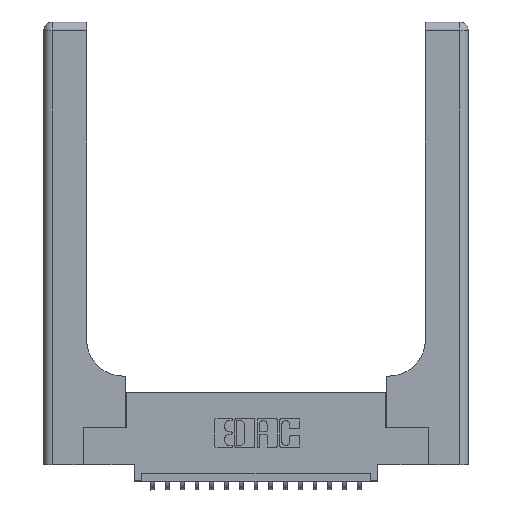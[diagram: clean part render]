
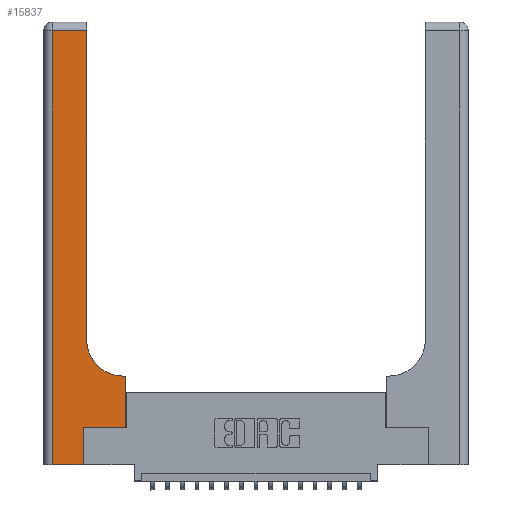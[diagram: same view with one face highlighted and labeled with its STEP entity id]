
A CAD part, top view. The second image highlights one B-rep face of the part: STEP entity #15837.
In plain terms, the highlighted planar face has unit normal (0, 0, 1).
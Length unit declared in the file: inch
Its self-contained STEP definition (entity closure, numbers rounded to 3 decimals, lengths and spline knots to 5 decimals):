
#398 = DIRECTION ( 'NONE',  ( -1., 0., 0. ) ) ;
#473 = EDGE_CURVE ( 'NONE', #16439, #4550, #7650, .T. ) ;
#478 = ORIENTED_EDGE ( 'NONE', *, *, #10949, .T. ) ;
#588 = VECTOR ( 'NONE', #18240, 39.37008 ) ;
#759 = VECTOR ( 'NONE', #15588, 39.37008 ) ;
#807 = ORIENTED_EDGE ( 'NONE', *, *, #1249, .T. ) ;
#1249 = EDGE_CURVE ( 'NONE', #12366, #1956, #19674, .T. ) ;
#1771 = AXIS2_PLACEMENT_3D ( 'NONE', #9812, #11354, #17633 ) ;
#1929 = CARTESIAN_POINT ( 'NONE',  ( 0.2915, 3., 0.37 ) ) ;
#1956 = VERTEX_POINT ( 'NONE', #12227 ) ;
#2508 = CARTESIAN_POINT ( 'NONE',  ( 0.5415, 0.6, 0.37 ) ) ;
#2827 = EDGE_CURVE ( 'NONE', #1956, #9334, #19178, .T. ) ;
#2902 = LINE ( 'NONE', #11200, #14275 ) ;
#3002 = CARTESIAN_POINT ( 'NONE',  ( 0.269, 0., 0.37 ) ) ;
#3038 = VERTEX_POINT ( 'NONE', #11050 ) ;
#3108 = ORIENTED_EDGE ( 'NONE', *, *, #2827, .T. ) ;
#3231 = VERTEX_POINT ( 'NONE', #3480 ) ;
#3290 = VECTOR ( 'NONE', #10494, 39.37008 ) ;
#3459 = LINE ( 'NONE', #1929, #15794 ) ;
#3480 = CARTESIAN_POINT ( 'NONE',  ( 0.2915, 2.94, 0.37 ) ) ;
#3725 = CARTESIAN_POINT ( 'NONE',  ( 0.269, 0., 0.37 ) ) ;
#3758 = ORIENTED_EDGE ( 'NONE', *, *, #8784, .T. ) ;
#4197 = VECTOR ( 'NONE', #13248, 39.37008 ) ;
#4314 = CARTESIAN_POINT ( 'NONE',  ( 0.5585, 0.6, 0.37 ) ) ;
#4550 = VERTEX_POINT ( 'NONE', #2508 ) ;
#5030 = DIRECTION ( 'NONE',  ( 0., 1., 0. ) ) ;
#5092 = FACE_OUTER_BOUND ( 'NONE', #13792, .T. ) ;
#5934 = CARTESIAN_POINT ( 'NONE',  ( 0.06, 0., 0.37 ) ) ;
#6849 = EDGE_CURVE ( 'NONE', #15107, #3231, #3459, .T. ) ;
#7074 = CARTESIAN_POINT ( 'NONE',  ( 0., 0., 0.37 ) ) ;
#7190 = EDGE_CURVE ( 'NONE', #9334, #16439, #17242, .T. ) ;
#7239 = DIRECTION ( 'NONE',  ( 0., 1., 0. ) ) ;
#7650 = LINE ( 'NONE', #16686, #588 ) ;
#7733 = CIRCLE ( 'NONE', #1771, 0.25 ) ;
#7760 = CARTESIAN_POINT ( 'NONE',  ( 0., 3., 0.37 ) ) ;
#8585 = CARTESIAN_POINT ( 'NONE',  ( 0.06, 3., 0.37 ) ) ;
#8784 = EDGE_CURVE ( 'NONE', #3231, #3038, #2902, .T. ) ;
#8812 = VECTOR ( 'NONE', #7239, 39.37008 ) ;
#9215 = CARTESIAN_POINT ( 'NONE',  ( 0.269, 0.25, 0.37 ) ) ;
#9264 = AXIS2_PLACEMENT_3D ( 'NONE', #7760, #17163, #14154 ) ;
#9334 = VERTEX_POINT ( 'NONE', #17503 ) ;
#9812 = CARTESIAN_POINT ( 'NONE',  ( 0.5415, 0.85, 0.37 ) ) ;
#10188 = ORIENTED_EDGE ( 'NONE', *, *, #17511, .T. ) ;
#10494 = DIRECTION ( 'NONE',  ( 1., 0., 0. ) ) ;
#10614 = VERTEX_POINT ( 'NONE', #5934 ) ;
#10949 = EDGE_CURVE ( 'NONE', #4550, #15107, #7733, .T. ) ;
#11050 = CARTESIAN_POINT ( 'NONE',  ( 0.06, 2.94, 0.37 ) ) ;
#11137 = LINE ( 'NONE', #7074, #3290 ) ;
#11166 = ORIENTED_EDGE ( 'NONE', *, *, #473, .T. ) ;
#11200 = CARTESIAN_POINT ( 'NONE',  ( 0., 2.94, 0.37 ) ) ;
#11322 = VECTOR ( 'NONE', #20113, 39.37008 ) ;
#11354 = DIRECTION ( 'NONE',  ( 0., 0., -1. ) ) ;
#11858 = EDGE_CURVE ( 'NONE', #10614, #12366, #11137, .T. ) ;
#12227 = CARTESIAN_POINT ( 'NONE',  ( 0.269, 0.25, 0.37 ) ) ;
#12366 = VERTEX_POINT ( 'NONE', #3725 ) ;
#12692 = ORIENTED_EDGE ( 'NONE', *, *, #6849, .T. ) ;
#13248 = DIRECTION ( 'NONE',  ( 0., -1., 0. ) ) ;
#13339 = LINE ( 'NONE', #8585, #4197 ) ;
#13792 = EDGE_LOOP ( 'NONE', ( #12692, #3758, #10188, #20191, #807, #3108, #15112, #11166, #478 ) ) ;
#14154 = DIRECTION ( 'NONE',  ( -1., 0., 0. ) ) ;
#14275 = VECTOR ( 'NONE', #398, 39.37008 ) ;
#15107 = VERTEX_POINT ( 'NONE', #15954 ) ;
#15112 = ORIENTED_EDGE ( 'NONE', *, *, #7190, .T. ) ;
#15588 = DIRECTION ( 'NONE',  ( 1., 0., 0. ) ) ;
#15644 = PLANE ( 'NONE',  #9264 ) ;
#15794 = VECTOR ( 'NONE', #5030, 39.37008 ) ;
#15837 = ADVANCED_FACE ( 'NONE', ( #5092 ), #15644, .F. ) ;
#15954 = CARTESIAN_POINT ( 'NONE',  ( 0.2915, 0.85, 0.37 ) ) ;
#16439 = VERTEX_POINT ( 'NONE', #4314 ) ;
#16686 = CARTESIAN_POINT ( 'NONE',  ( 0.2915, 0.6, 0.37 ) ) ;
#16717 = CARTESIAN_POINT ( 'NONE',  ( 0.5585, 0.25, 0.37 ) ) ;
#17163 = DIRECTION ( 'NONE',  ( 0., 0., -1. ) ) ;
#17242 = LINE ( 'NONE', #16717, #8812 ) ;
#17503 = CARTESIAN_POINT ( 'NONE',  ( 0.5585, 0.25, 0.37 ) ) ;
#17511 = EDGE_CURVE ( 'NONE', #3038, #10614, #13339, .T. ) ;
#17633 = DIRECTION ( 'NONE',  ( 1., 0., 0. ) ) ;
#18240 = DIRECTION ( 'NONE',  ( -1., 0., 0. ) ) ;
#19178 = LINE ( 'NONE', #9215, #759 ) ;
#19674 = LINE ( 'NONE', #3002, #11322 ) ;
#20113 = DIRECTION ( 'NONE',  ( 0., 1., 0. ) ) ;
#20191 = ORIENTED_EDGE ( 'NONE', *, *, #11858, .T. ) ;
